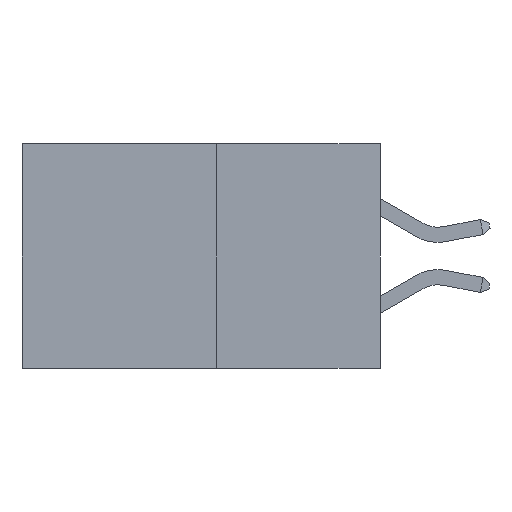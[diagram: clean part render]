
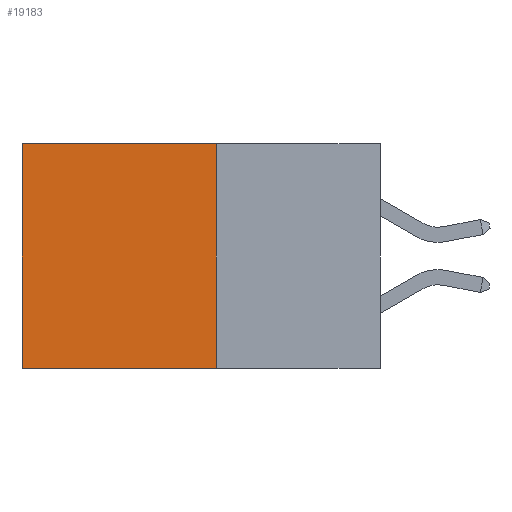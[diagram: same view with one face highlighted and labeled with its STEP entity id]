
A CAD part, left-side view. The second image highlights one B-rep face of the part: STEP entity #19183.
In plain terms, the highlighted planar face has unit normal (-1, 0, 0).
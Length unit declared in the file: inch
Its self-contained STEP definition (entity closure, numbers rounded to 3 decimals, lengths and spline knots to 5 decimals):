
#992 = ORIENTED_EDGE ( 'NONE', *, *, #8897, .F. ) ;
#1033 = VERTEX_POINT ( 'NONE', #19567 ) ;
#1988 = CARTESIAN_POINT ( 'NONE',  ( 0.277, 0.27, -0.37 ) ) ;
#2470 = CARTESIAN_POINT ( 'NONE',  ( 0.277, 0.59, 0. ) ) ;
#2724 = FACE_OUTER_BOUND ( 'NONE', #29761, .T. ) ;
#4658 = DIRECTION ( 'NONE',  ( 1., 0., 0. ) ) ;
#5069 = VERTEX_POINT ( 'NONE', #22010 ) ;
#5416 = VECTOR ( 'NONE', #16721, 39.37008 ) ;
#6202 = VECTOR ( 'NONE', #13817, 39.37008 ) ;
#6272 = LINE ( 'NONE', #15852, #33272 ) ;
#6320 = EDGE_CURVE ( 'NONE', #5069, #31708, #6272, .T. ) ;
#8897 = EDGE_CURVE ( 'NONE', #29639, #1033, #19442, .T. ) ;
#9901 = AXIS2_PLACEMENT_3D ( 'NONE', #1988, #4658, #23036 ) ;
#11146 = CARTESIAN_POINT ( 'NONE',  ( 0.277, 0.59, -0.37 ) ) ;
#11451 = EDGE_CURVE ( 'NONE', #5069, #29639, #24922, .T. ) ;
#11786 = CARTESIAN_POINT ( 'NONE',  ( 0.277, 0.27, -0.37 ) ) ;
#11993 = ORIENTED_EDGE ( 'NONE', *, *, #11451, .F. ) ;
#13817 = DIRECTION ( 'NONE',  ( 0., 0., -1. ) ) ;
#15852 = CARTESIAN_POINT ( 'NONE',  ( 0.277, 0.27, 0. ) ) ;
#16721 = DIRECTION ( 'NONE',  ( 0., 1., 0. ) ) ;
#17843 = PLANE ( 'NONE',  #9901 ) ;
#19183 = ADVANCED_FACE ( 'NONE', ( #2724 ), #17843, .F. ) ;
#19340 = CARTESIAN_POINT ( 'NONE',  ( 0.277, 0.27, -0.37 ) ) ;
#19442 = LINE ( 'NONE', #19340, #5416 ) ;
#19567 = CARTESIAN_POINT ( 'NONE',  ( 0.277, 0.59, -0.37 ) ) ;
#20436 = ORIENTED_EDGE ( 'NONE', *, *, #31898, .T. ) ;
#20953 = DIRECTION ( 'NONE',  ( 0., 1., 0. ) ) ;
#22010 = CARTESIAN_POINT ( 'NONE',  ( 0.277, 0.27, 0. ) ) ;
#23036 = DIRECTION ( 'NONE',  ( 0., 0., -1. ) ) ;
#24922 = LINE ( 'NONE', #28864, #31036 ) ;
#25446 = LINE ( 'NONE', #11146, #6202 ) ;
#27660 = ORIENTED_EDGE ( 'NONE', *, *, #6320, .T. ) ;
#28864 = CARTESIAN_POINT ( 'NONE',  ( 0.277, 0.27, -0.37 ) ) ;
#29639 = VERTEX_POINT ( 'NONE', #11786 ) ;
#29761 = EDGE_LOOP ( 'NONE', ( #20436, #992, #11993, #27660 ) ) ;
#31036 = VECTOR ( 'NONE', #31479, 39.37008 ) ;
#31479 = DIRECTION ( 'NONE',  ( 0., 0., -1. ) ) ;
#31708 = VERTEX_POINT ( 'NONE', #2470 ) ;
#31898 = EDGE_CURVE ( 'NONE', #31708, #1033, #25446, .T. ) ;
#33272 = VECTOR ( 'NONE', #20953, 39.37008 ) ;
